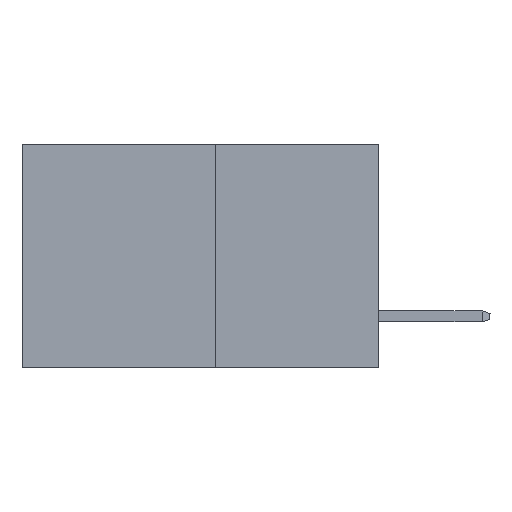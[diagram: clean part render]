
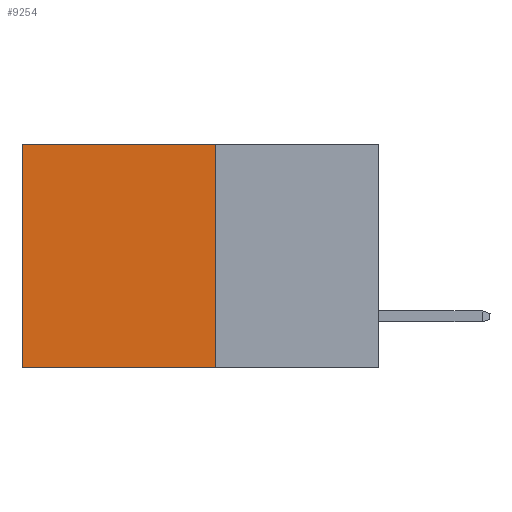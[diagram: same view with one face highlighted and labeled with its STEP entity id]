
A CAD part, left-side view. The second image highlights one B-rep face of the part: STEP entity #9254.
In plain terms, the highlighted planar face has unit normal (-1, 0, 0).
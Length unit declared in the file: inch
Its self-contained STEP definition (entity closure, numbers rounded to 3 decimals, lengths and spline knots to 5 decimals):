
#137 = LINE ( 'NONE', #8037, #6064 ) ;
#183 = EDGE_CURVE ( 'NONE', #6584, #655, #3981, .T. ) ;
#392 = DIRECTION ( 'NONE',  ( 0., 0., -1. ) ) ;
#655 = VERTEX_POINT ( 'NONE', #4684 ) ;
#719 = CARTESIAN_POINT ( 'NONE',  ( 0.277, 0.59, -0.37 ) ) ;
#987 = DIRECTION ( 'NONE',  ( 0., 0., -1. ) ) ;
#1016 = EDGE_CURVE ( 'NONE', #655, #5388, #8354, .T. ) ;
#1055 = PLANE ( 'NONE',  #5145 ) ;
#1141 = CARTESIAN_POINT ( 'NONE',  ( 0.277, 0.27, -0.37 ) ) ;
#1429 = DIRECTION ( 'NONE',  ( 1., 0., 0. ) ) ;
#1509 = VECTOR ( 'NONE', #5465, 39.37008 ) ;
#1564 = CARTESIAN_POINT ( 'NONE',  ( 0.277, 0.27, -0.37 ) ) ;
#1670 = VERTEX_POINT ( 'NONE', #1564 ) ;
#1703 = VECTOR ( 'NONE', #6447, 39.37008 ) ;
#1840 = EDGE_CURVE ( 'NONE', #6584, #1670, #137, .T. ) ;
#1900 = EDGE_CURVE ( 'NONE', #1670, #5388, #9108, .T. ) ;
#2302 = ORIENTED_EDGE ( 'NONE', *, *, #1016, .T. ) ;
#2354 = ORIENTED_EDGE ( 'NONE', *, *, #1900, .F. ) ;
#2518 = ORIENTED_EDGE ( 'NONE', *, *, #1840, .F. ) ;
#2544 = ORIENTED_EDGE ( 'NONE', *, *, #183, .T. ) ;
#3981 = LINE ( 'NONE', #7343, #1703 ) ;
#4089 = EDGE_LOOP ( 'NONE', ( #2302, #2354, #2518, #2544 ) ) ;
#4584 = CARTESIAN_POINT ( 'NONE',  ( 0.277, 0.27, 0. ) ) ;
#4684 = CARTESIAN_POINT ( 'NONE',  ( 0.277, 0.59, 0. ) ) ;
#5145 = AXIS2_PLACEMENT_3D ( 'NONE', #1141, #1429, #987 ) ;
#5388 = VERTEX_POINT ( 'NONE', #719 ) ;
#5465 = DIRECTION ( 'NONE',  ( 0., 1., 0. ) ) ;
#6064 = VECTOR ( 'NONE', #392, 39.37008 ) ;
#6301 = DIRECTION ( 'NONE',  ( 0., 0., -1. ) ) ;
#6313 = CARTESIAN_POINT ( 'NONE',  ( 0.277, 0.59, -0.37 ) ) ;
#6447 = DIRECTION ( 'NONE',  ( 0., 1., 0. ) ) ;
#6584 = VERTEX_POINT ( 'NONE', #4584 ) ;
#7343 = CARTESIAN_POINT ( 'NONE',  ( 0.277, 0.27, 0. ) ) ;
#8037 = CARTESIAN_POINT ( 'NONE',  ( 0.277, 0.27, -0.37 ) ) ;
#8143 = VECTOR ( 'NONE', #6301, 39.37008 ) ;
#8354 = LINE ( 'NONE', #6313, #8143 ) ;
#8659 = FACE_OUTER_BOUND ( 'NONE', #4089, .T. ) ;
#8869 = CARTESIAN_POINT ( 'NONE',  ( 0.277, 0.27, -0.37 ) ) ;
#9108 = LINE ( 'NONE', #8869, #1509 ) ;
#9254 = ADVANCED_FACE ( 'NONE', ( #8659 ), #1055, .F. ) ;
